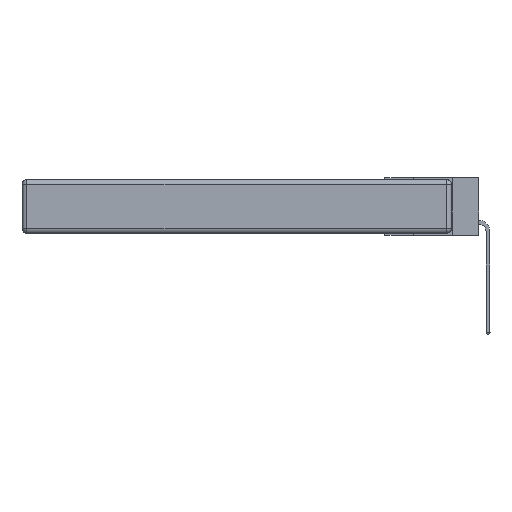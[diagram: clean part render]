
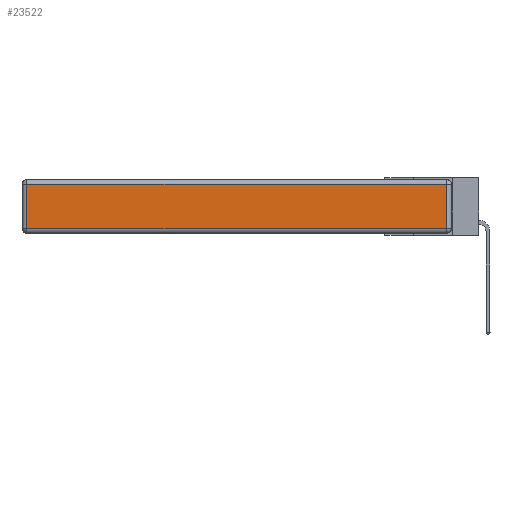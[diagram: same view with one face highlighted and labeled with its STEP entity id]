
A CAD part, left-side view. The second image highlights one B-rep face of the part: STEP entity #23522.
In plain terms, the highlighted planar face has unit normal (-1, 0, 0).
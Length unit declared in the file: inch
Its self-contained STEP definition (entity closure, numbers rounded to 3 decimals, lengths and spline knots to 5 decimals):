
#212 = CARTESIAN_POINT ( 'NONE',  ( 0., 2.72, -0.343 ) ) ;
#1601 = LINE ( 'NONE', #212, #7953 ) ;
#1868 = EDGE_LOOP ( 'NONE', ( #3305, #8216, #10911, #2137 ) ) ;
#1951 = CARTESIAN_POINT ( 'NONE',  ( 0., 0.03, -0.03 ) ) ;
#2089 = EDGE_CURVE ( 'NONE', #7022, #12540, #7766, .T. ) ;
#2137 = ORIENTED_EDGE ( 'NONE', *, *, #23784, .T. ) ;
#2490 = DIRECTION ( 'NONE',  ( 0., 1., 0. ) ) ;
#2741 = EDGE_CURVE ( 'NONE', #13110, #13271, #5718, .T. ) ;
#2857 = VECTOR ( 'NONE', #12231, 39.37008 ) ;
#3237 = DIRECTION ( 'NONE',  ( 0., 0., 1. ) ) ;
#3261 = LINE ( 'NONE', #19336, #14721 ) ;
#3305 = ORIENTED_EDGE ( 'NONE', *, *, #2089, .T. ) ;
#3781 = CARTESIAN_POINT ( 'NONE',  ( 0., 2.72, -0.313 ) ) ;
#5718 = LINE ( 'NONE', #6301, #15726 ) ;
#6235 = CARTESIAN_POINT ( 'NONE',  ( 0., 0., -0.313 ) ) ;
#6301 = CARTESIAN_POINT ( 'NONE',  ( 0., 2.75, -0.03 ) ) ;
#7022 = VERTEX_POINT ( 'NONE', #3781 ) ;
#7766 = LINE ( 'NONE', #6235, #2857 ) ;
#7953 = VECTOR ( 'NONE', #20200, 39.37008 ) ;
#8216 = ORIENTED_EDGE ( 'NONE', *, *, #16825, .T. ) ;
#8935 = DIRECTION ( 'NONE',  ( -1., 0., 0. ) ) ;
#10322 = CARTESIAN_POINT ( 'NONE',  ( 0., 2.72, -0.03 ) ) ;
#10911 = ORIENTED_EDGE ( 'NONE', *, *, #2741, .T. ) ;
#12231 = DIRECTION ( 'NONE',  ( 0., -1., 0. ) ) ;
#12540 = VERTEX_POINT ( 'NONE', #14566 ) ;
#12683 = CARTESIAN_POINT ( 'NONE',  ( 0., 0., -0.343 ) ) ;
#13110 = VERTEX_POINT ( 'NONE', #1951 ) ;
#13271 = VERTEX_POINT ( 'NONE', #10322 ) ;
#14566 = CARTESIAN_POINT ( 'NONE',  ( 0., 0.03, -0.313 ) ) ;
#14721 = VECTOR ( 'NONE', #19108, 39.37008 ) ;
#15726 = VECTOR ( 'NONE', #2490, 39.37008 ) ;
#16825 = EDGE_CURVE ( 'NONE', #12540, #13110, #3261, .T. ) ;
#19108 = DIRECTION ( 'NONE',  ( 0., 0., 1. ) ) ;
#19290 = AXIS2_PLACEMENT_3D ( 'NONE', #12683, #8935, #3237 ) ;
#19336 = CARTESIAN_POINT ( 'NONE',  ( 0., 0.03, -0.343 ) ) ;
#19780 = PLANE ( 'NONE',  #19290 ) ;
#20200 = DIRECTION ( 'NONE',  ( 0., 0., -1. ) ) ;
#22536 = FACE_OUTER_BOUND ( 'NONE', #1868, .T. ) ;
#23522 = ADVANCED_FACE ( 'NONE', ( #22536 ), #19780, .T. ) ;
#23784 = EDGE_CURVE ( 'NONE', #13271, #7022, #1601, .T. ) ;
